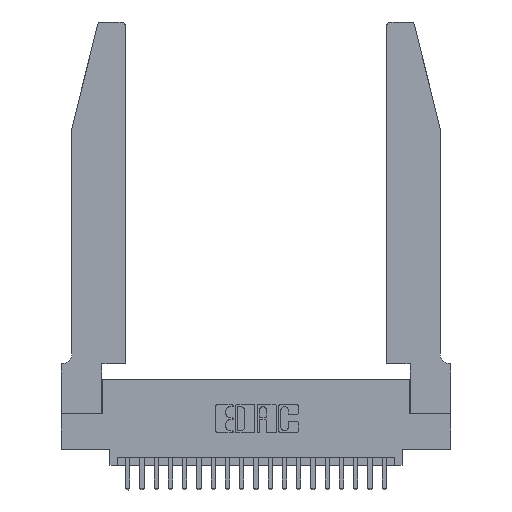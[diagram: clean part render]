
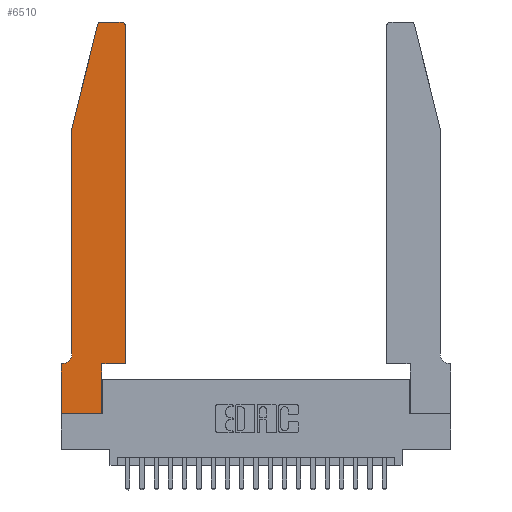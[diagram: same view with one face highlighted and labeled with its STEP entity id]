
A CAD part, top view. The second image highlights one B-rep face of the part: STEP entity #6510.
In plain terms, the highlighted planar face has unit normal (0, 0, 1).
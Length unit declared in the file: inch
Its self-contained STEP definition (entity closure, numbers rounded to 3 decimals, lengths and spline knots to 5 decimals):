
#11 = EDGE_CURVE ( 'NONE', #20481, #2120, #22121, .T. ) ;
#153 = CIRCLE ( 'NONE', #15243, 0.07 ) ;
#202 = EDGE_CURVE ( 'NONE', #20648, #9348, #153, .T. ) ;
#206 = ORIENTED_EDGE ( 'NONE', *, *, #10393, .T. ) ;
#273 = CARTESIAN_POINT ( 'NONE',  ( 0.4205, 2.72, 0.37 ) ) ;
#376 = EDGE_CURVE ( 'NONE', #10692, #9251, #12962, .T. ) ;
#686 = CARTESIAN_POINT ( 'NONE',  ( 0.0755, 2., 0.37 ) ) ;
#1005 = CARTESIAN_POINT ( 'NONE',  ( 0.4205, 2.75, 0.37 ) ) ;
#1088 = CARTESIAN_POINT ( 'NONE',  ( 0.4505, 0.35, 0.37 ) ) ;
#1781 = CIRCLE ( 'NONE', #3267, 0.03 ) ;
#1925 = CARTESIAN_POINT ( 'NONE',  ( 0.4505, 2.72, 0.37 ) ) ;
#1931 = ORIENTED_EDGE ( 'NONE', *, *, #8043, .T. ) ;
#2057 = VERTEX_POINT ( 'NONE', #2816 ) ;
#2120 = VERTEX_POINT ( 'NONE', #4643 ) ;
#2488 = EDGE_CURVE ( 'NONE', #2120, #6160, #11269, .T. ) ;
#2526 = VECTOR ( 'NONE', #18635, 39.37008 ) ;
#2635 = EDGE_CURVE ( 'NONE', #2057, #20481, #10697, .T. ) ;
#2789 = CARTESIAN_POINT ( 'NONE',  ( 0.4505, 0.35, 0.37 ) ) ;
#2816 = CARTESIAN_POINT ( 'NONE',  ( 0., 0.35, 0.37 ) ) ;
#3267 = AXIS2_PLACEMENT_3D ( 'NONE', #273, #3855, #7507 ) ;
#3297 = CARTESIAN_POINT ( 'NONE',  ( 0.4505, 0.35, 0.37 ) ) ;
#3422 = CARTESIAN_POINT ( 'NONE',  ( 0.0755, 0.35, 0.37 ) ) ;
#3547 = CARTESIAN_POINT ( 'NONE',  ( 0., 0.35, 0.37 ) ) ;
#3609 = VECTOR ( 'NONE', #15934, 39.37008 ) ;
#3632 = LINE ( 'NONE', #3422, #21960 ) ;
#3665 = LINE ( 'NONE', #1088, #2526 ) ;
#3855 = DIRECTION ( 'NONE',  ( 0., 0., 1. ) ) ;
#4560 = ORIENTED_EDGE ( 'NONE', *, *, #2635, .T. ) ;
#4643 = CARTESIAN_POINT ( 'NONE',  ( 0.2865, 0., 0.37 ) ) ;
#4804 = VECTOR ( 'NONE', #22709, 39.37008 ) ;
#5103 = CARTESIAN_POINT ( 'NONE',  ( 0., 0., 0.37 ) ) ;
#5569 = DIRECTION ( 'NONE',  ( 0., -1., 0. ) ) ;
#5824 = ORIENTED_EDGE ( 'NONE', *, *, #6339, .T. ) ;
#5963 = CARTESIAN_POINT ( 'NONE',  ( 0.2865, 0.35, 0.37 ) ) ;
#6160 = VERTEX_POINT ( 'NONE', #5963 ) ;
#6339 = EDGE_CURVE ( 'NONE', #7174, #7811, #1781, .T. ) ;
#6355 = DIRECTION ( 'NONE',  ( 0., 1., 0. ) ) ;
#6510 = ADVANCED_FACE ( 'NONE', ( #15702 ), #10589, .T. ) ;
#7059 = CARTESIAN_POINT ( 'NONE',  ( 0.284, 2.72, 0.37 ) ) ;
#7174 = VERTEX_POINT ( 'NONE', #1925 ) ;
#7507 = DIRECTION ( 'NONE',  ( 1., 0., 0. ) ) ;
#7668 = ORIENTED_EDGE ( 'NONE', *, *, #7972, .T. ) ;
#7811 = VERTEX_POINT ( 'NONE', #1005 ) ;
#7871 = ORIENTED_EDGE ( 'NONE', *, *, #11, .T. ) ;
#7972 = EDGE_CURVE ( 'NONE', #15122, #10692, #10937, .T. ) ;
#8038 = CARTESIAN_POINT ( 'NONE',  ( 0.0055, 0.42, 0.37 ) ) ;
#8043 = EDGE_CURVE ( 'NONE', #6160, #15791, #3665, .T. ) ;
#8155 = VECTOR ( 'NONE', #10809, 39.37008 ) ;
#8343 = LINE ( 'NONE', #12313, #3609 ) ;
#8788 = EDGE_CURVE ( 'NONE', #9251, #20648, #11986, .T. ) ;
#8903 = CARTESIAN_POINT ( 'NONE',  ( 0.0055, 0.35, 0.37 ) ) ;
#8936 = CARTESIAN_POINT ( 'NONE',  ( 0., 0., 0.37 ) ) ;
#8947 = AXIS2_PLACEMENT_3D ( 'NONE', #3547, #17809, #10811 ) ;
#9222 = ORIENTED_EDGE ( 'NONE', *, *, #8788, .T. ) ;
#9251 = VERTEX_POINT ( 'NONE', #22620 ) ;
#9348 = VERTEX_POINT ( 'NONE', #8903 ) ;
#9470 = CARTESIAN_POINT ( 'NONE',  ( 0.0755, 0.42, 0.37 ) ) ;
#10124 = ORIENTED_EDGE ( 'NONE', *, *, #376, .T. ) ;
#10393 = EDGE_CURVE ( 'NONE', #7811, #15122, #8343, .T. ) ;
#10544 = DIRECTION ( 'NONE',  ( -1., 0., 0. ) ) ;
#10589 = PLANE ( 'NONE',  #8947 ) ;
#10692 = VERTEX_POINT ( 'NONE', #19848 ) ;
#10697 = LINE ( 'NONE', #8936, #8155 ) ;
#10809 = DIRECTION ( 'NONE',  ( 0., -1., 0. ) ) ;
#10811 = DIRECTION ( 'NONE',  ( 1., 0., 0. ) ) ;
#10937 = CIRCLE ( 'NONE', #14312, 0.03 ) ;
#10987 = DIRECTION ( 'NONE',  ( 1., 0., 0. ) ) ;
#11269 = LINE ( 'NONE', #12040, #4804 ) ;
#11332 = VECTOR ( 'NONE', #13481, 39.37008 ) ;
#11405 = DIRECTION ( 'NONE',  ( -1., 0., 0. ) ) ;
#11597 = ORIENTED_EDGE ( 'NONE', *, *, #17108, .T. ) ;
#11602 = CARTESIAN_POINT ( 'NONE',  ( 0.284, 2.75, 0.37 ) ) ;
#11986 = LINE ( 'NONE', #686, #18900 ) ;
#12040 = CARTESIAN_POINT ( 'NONE',  ( 0.2865, 0.35, 0.37 ) ) ;
#12313 = CARTESIAN_POINT ( 'NONE',  ( 0.2605, 2.75, 0.37 ) ) ;
#12506 = DIRECTION ( 'NONE',  ( 0., 0., 1. ) ) ;
#12962 = LINE ( 'NONE', #18558, #11332 ) ;
#12998 = DIRECTION ( 'NONE',  ( 0., 0., -1. ) ) ;
#13481 = DIRECTION ( 'NONE',  ( -0.239, -0.971, 0. ) ) ;
#14312 = AXIS2_PLACEMENT_3D ( 'NONE', #7059, #12506, #21777 ) ;
#14316 = ORIENTED_EDGE ( 'NONE', *, *, #2488, .T. ) ;
#15122 = VERTEX_POINT ( 'NONE', #11602 ) ;
#15243 = AXIS2_PLACEMENT_3D ( 'NONE', #8038, #12998, #11405 ) ;
#15702 = FACE_OUTER_BOUND ( 'NONE', #21062, .T. ) ;
#15791 = VERTEX_POINT ( 'NONE', #3297 ) ;
#15934 = DIRECTION ( 'NONE',  ( -1., 0., 0. ) ) ;
#16228 = EDGE_CURVE ( 'NONE', #15791, #7174, #21450, .T. ) ;
#16364 = CARTESIAN_POINT ( 'NONE',  ( 0., 0., 0.37 ) ) ;
#17108 = EDGE_CURVE ( 'NONE', #9348, #2057, #3632, .T. ) ;
#17809 = DIRECTION ( 'NONE',  ( 0., 0., 1. ) ) ;
#18558 = CARTESIAN_POINT ( 'NONE',  ( 0.0755, 2., 0.37 ) ) ;
#18635 = DIRECTION ( 'NONE',  ( 1., 0., 0. ) ) ;
#18900 = VECTOR ( 'NONE', #5569, 39.37008 ) ;
#18950 = ORIENTED_EDGE ( 'NONE', *, *, #16228, .T. ) ;
#19780 = ORIENTED_EDGE ( 'NONE', *, *, #202, .T. ) ;
#19848 = CARTESIAN_POINT ( 'NONE',  ( 0.25487, 2.72718, 0.37 ) ) ;
#20481 = VERTEX_POINT ( 'NONE', #5103 ) ;
#20648 = VERTEX_POINT ( 'NONE', #9470 ) ;
#21062 = EDGE_LOOP ( 'NONE', ( #206, #7668, #10124, #9222, #19780, #11597, #4560, #7871, #14316, #1931, #18950, #5824 ) ) ;
#21450 = LINE ( 'NONE', #2789, #21987 ) ;
#21777 = DIRECTION ( 'NONE',  ( 1., 0., 0. ) ) ;
#21855 = VECTOR ( 'NONE', #10987, 39.37008 ) ;
#21960 = VECTOR ( 'NONE', #10544, 39.37008 ) ;
#21987 = VECTOR ( 'NONE', #6355, 39.37008 ) ;
#22121 = LINE ( 'NONE', #16364, #21855 ) ;
#22620 = CARTESIAN_POINT ( 'NONE',  ( 0.0755, 2., 0.37 ) ) ;
#22709 = DIRECTION ( 'NONE',  ( 0., 1., 0. ) ) ;
